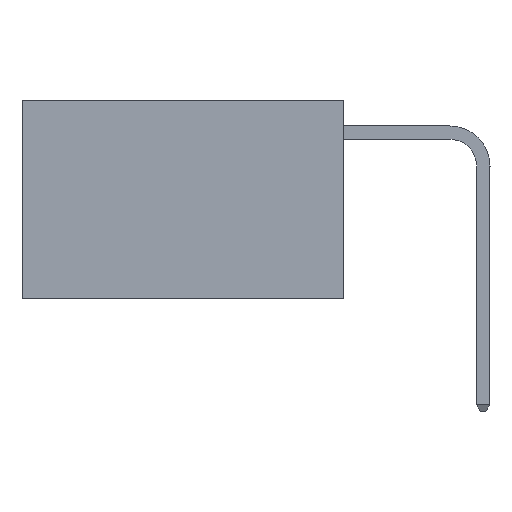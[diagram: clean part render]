
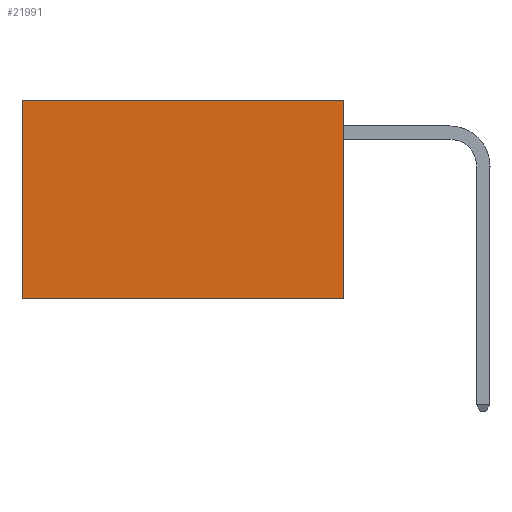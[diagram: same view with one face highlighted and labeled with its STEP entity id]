
A CAD part, left-side view. The second image highlights one B-rep face of the part: STEP entity #21991.
In plain terms, the highlighted planar face has unit normal (-1, 0, 0).
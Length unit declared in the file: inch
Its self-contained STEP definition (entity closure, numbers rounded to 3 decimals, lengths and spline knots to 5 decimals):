
#2114 = CARTESIAN_POINT ( 'NONE',  ( 0.2625, 0., 0. ) ) ;
#2675 = LINE ( 'NONE', #2114, #7030 ) ;
#3173 = EDGE_CURVE ( 'NONE', #9168, #13895, #11736, .T. ) ;
#3214 = VERTEX_POINT ( 'NONE', #5477 ) ;
#3528 = CARTESIAN_POINT ( 'NONE',  ( 0.2625, 0.6, 0. ) ) ;
#5023 = ORIENTED_EDGE ( 'NONE', *, *, #13448, .F. ) ;
#5389 = DIRECTION ( 'NONE',  ( 0., 0., -1. ) ) ;
#5477 = CARTESIAN_POINT ( 'NONE',  ( 0.2625, 0., 0. ) ) ;
#6226 = DIRECTION ( 'NONE',  ( 1., 0., 0. ) ) ;
#6822 = ORIENTED_EDGE ( 'NONE', *, *, #21281, .F. ) ;
#7030 = VECTOR ( 'NONE', #13347, 39.37008 ) ;
#9168 = VERTEX_POINT ( 'NONE', #19464 ) ;
#9828 = CARTESIAN_POINT ( 'NONE',  ( 0.2625, 0., 0. ) ) ;
#9831 = DIRECTION ( 'NONE',  ( 0., 1., 0. ) ) ;
#11012 = VECTOR ( 'NONE', #9831, 39.37008 ) ;
#11700 = DIRECTION ( 'NONE',  ( 0., 0., -1. ) ) ;
#11736 = LINE ( 'NONE', #3528, #20960 ) ;
#11757 = PLANE ( 'NONE',  #18962 ) ;
#12131 = CARTESIAN_POINT ( 'NONE',  ( 0.2625, 0., -0.37 ) ) ;
#13347 = DIRECTION ( 'NONE',  ( 0., 1., 0. ) ) ;
#13448 = EDGE_CURVE ( 'NONE', #3214, #20809, #13487, .T. ) ;
#13487 = LINE ( 'NONE', #9828, #22666 ) ;
#13895 = VERTEX_POINT ( 'NONE', #18788 ) ;
#15950 = LINE ( 'NONE', #19051, #11012 ) ;
#15978 = ORIENTED_EDGE ( 'NONE', *, *, #3173, .T. ) ;
#17324 = CARTESIAN_POINT ( 'NONE',  ( 0.2625, 0., 0. ) ) ;
#18788 = CARTESIAN_POINT ( 'NONE',  ( 0.2625, 0.6, -0.37 ) ) ;
#18962 = AXIS2_PLACEMENT_3D ( 'NONE', #17324, #6226, #19180 ) ;
#19051 = CARTESIAN_POINT ( 'NONE',  ( 0.2625, 0., -0.37 ) ) ;
#19180 = DIRECTION ( 'NONE',  ( 0., 0., -1. ) ) ;
#19370 = FACE_OUTER_BOUND ( 'NONE', #21232, .T. ) ;
#19464 = CARTESIAN_POINT ( 'NONE',  ( 0.2625, 0.6, 0. ) ) ;
#19761 = EDGE_CURVE ( 'NONE', #3214, #9168, #2675, .T. ) ;
#20809 = VERTEX_POINT ( 'NONE', #12131 ) ;
#20960 = VECTOR ( 'NONE', #5389, 39.37008 ) ;
#21232 = EDGE_LOOP ( 'NONE', ( #15978, #6822, #5023, #23211 ) ) ;
#21281 = EDGE_CURVE ( 'NONE', #20809, #13895, #15950, .T. ) ;
#21991 = ADVANCED_FACE ( 'NONE', ( #19370 ), #11757, .F. ) ;
#22666 = VECTOR ( 'NONE', #11700, 39.37008 ) ;
#23211 = ORIENTED_EDGE ( 'NONE', *, *, #19761, .T. ) ;
